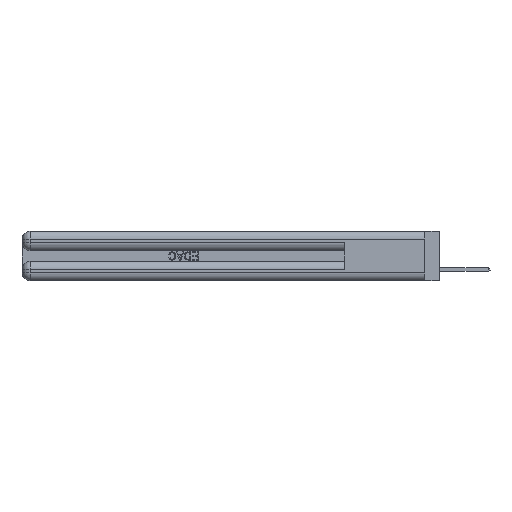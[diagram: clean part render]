
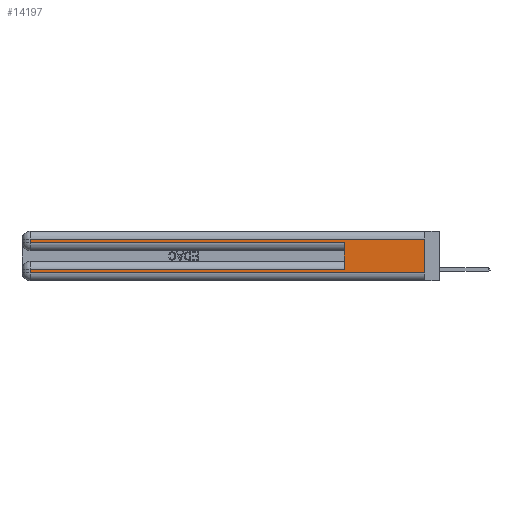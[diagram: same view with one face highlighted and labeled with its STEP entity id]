
A CAD part, left-side view. The second image highlights one B-rep face of the part: STEP entity #14197.
In plain terms, the highlighted planar face has unit normal (-1, 0, 0).
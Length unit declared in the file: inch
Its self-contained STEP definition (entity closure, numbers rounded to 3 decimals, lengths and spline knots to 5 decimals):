
#146 = EDGE_CURVE ( 'NONE', #34508, #25127, #3830, .T. ) ;
#267 = FACE_OUTER_BOUND ( 'NONE', #14080, .T. ) ;
#1153 = EDGE_CURVE ( 'NONE', #34851, #18567, #18973, .T. ) ;
#1823 = CARTESIAN_POINT ( 'NONE',  ( 0., 0., 0.31 ) ) ;
#2283 = CARTESIAN_POINT ( 'NONE',  ( 0., 0., 0.37 ) ) ;
#3098 = CARTESIAN_POINT ( 'NONE',  ( 0., 2.94, 0.06 ) ) ;
#3830 = LINE ( 'NONE', #24998, #38148 ) ;
#3988 = LINE ( 'NONE', #23489, #22519 ) ;
#4691 = ORIENTED_EDGE ( 'NONE', *, *, #10071, .T. ) ;
#5252 = VECTOR ( 'NONE', #17606, 39.37008 ) ;
#5422 = LINE ( 'NONE', #22631, #32078 ) ;
#6805 = CARTESIAN_POINT ( 'NONE',  ( 0., 0., 0.06 ) ) ;
#6834 = CARTESIAN_POINT ( 'NONE',  ( 0., 0., 0.37 ) ) ;
#7089 = LINE ( 'NONE', #20087, #37565 ) ;
#7390 = VERTEX_POINT ( 'NONE', #17802 ) ;
#8117 = DIRECTION ( 'NONE',  ( 0., 0., -1. ) ) ;
#8640 = ORIENTED_EDGE ( 'NONE', *, *, #18666, .F. ) ;
#10043 = VERTEX_POINT ( 'NONE', #35858 ) ;
#10071 = EDGE_CURVE ( 'NONE', #25127, #26792, #26643, .T. ) ;
#11554 = ORIENTED_EDGE ( 'NONE', *, *, #20790, .T. ) ;
#12254 = VERTEX_POINT ( 'NONE', #19260 ) ;
#12385 = CARTESIAN_POINT ( 'NONE',  ( 0., 2.94, 0.285 ) ) ;
#13328 = DIRECTION ( 'NONE',  ( 0., 1., 0. ) ) ;
#14080 = EDGE_LOOP ( 'NONE', ( #8640, #29875, #4691, #33569, #20254, #11554, #17339, #21712 ) ) ;
#14197 = ADVANCED_FACE ( 'NONE', ( #267 ), #20209, .F. ) ;
#17339 = ORIENTED_EDGE ( 'NONE', *, *, #24654, .T. ) ;
#17606 = DIRECTION ( 'NONE',  ( 0., 0., -1. ) ) ;
#17802 = CARTESIAN_POINT ( 'NONE',  ( 0., 0.6, 0.285 ) ) ;
#17845 = CARTESIAN_POINT ( 'NONE',  ( 0., 0., 0.085 ) ) ;
#18298 = VECTOR ( 'NONE', #38304, 39.37008 ) ;
#18567 = VERTEX_POINT ( 'NONE', #6805 ) ;
#18593 = DIRECTION ( 'NONE',  ( 0., 0., -1. ) ) ;
#18666 = EDGE_CURVE ( 'NONE', #34508, #18567, #25720, .T. ) ;
#18973 = LINE ( 'NONE', #37427, #21849 ) ;
#19260 = CARTESIAN_POINT ( 'NONE',  ( 0., 0.6, 0.085 ) ) ;
#19710 = DIRECTION ( 'NONE',  ( 0., 0., 1. ) ) ;
#20087 = CARTESIAN_POINT ( 'NONE',  ( 0., 2.94, 0.37 ) ) ;
#20209 = PLANE ( 'NONE',  #24529 ) ;
#20254 = ORIENTED_EDGE ( 'NONE', *, *, #37326, .F. ) ;
#20790 = EDGE_CURVE ( 'NONE', #12254, #10043, #26467, .T. ) ;
#21712 = ORIENTED_EDGE ( 'NONE', *, *, #1153, .T. ) ;
#21832 = VECTOR ( 'NONE', #18593, 39.37008 ) ;
#21849 = VECTOR ( 'NONE', #34229, 39.37008 ) ;
#22519 = VECTOR ( 'NONE', #35354, 39.37008 ) ;
#22631 = CARTESIAN_POINT ( 'NONE',  ( 0., 0.6, 0.145 ) ) ;
#23489 = CARTESIAN_POINT ( 'NONE',  ( 0., 0., 0.285 ) ) ;
#24529 = AXIS2_PLACEMENT_3D ( 'NONE', #2283, #38726, #8117 ) ;
#24654 = EDGE_CURVE ( 'NONE', #10043, #34851, #7089, .T. ) ;
#24998 = CARTESIAN_POINT ( 'NONE',  ( 0., 0., 0.31 ) ) ;
#25127 = VERTEX_POINT ( 'NONE', #26168 ) ;
#25720 = LINE ( 'NONE', #6834, #21832 ) ;
#26168 = CARTESIAN_POINT ( 'NONE',  ( 0., 2.94, 0.31 ) ) ;
#26467 = LINE ( 'NONE', #17845, #18298 ) ;
#26643 = LINE ( 'NONE', #38523, #5252 ) ;
#26792 = VERTEX_POINT ( 'NONE', #12385 ) ;
#28453 = EDGE_CURVE ( 'NONE', #26792, #7390, #3988, .T. ) ;
#29875 = ORIENTED_EDGE ( 'NONE', *, *, #146, .T. ) ;
#32078 = VECTOR ( 'NONE', #19710, 39.37008 ) ;
#33569 = ORIENTED_EDGE ( 'NONE', *, *, #28453, .T. ) ;
#34229 = DIRECTION ( 'NONE',  ( 0., -1., 0. ) ) ;
#34508 = VERTEX_POINT ( 'NONE', #1823 ) ;
#34851 = VERTEX_POINT ( 'NONE', #3098 ) ;
#35354 = DIRECTION ( 'NONE',  ( 0., -1., 0. ) ) ;
#35670 = DIRECTION ( 'NONE',  ( 0., 0., -1. ) ) ;
#35858 = CARTESIAN_POINT ( 'NONE',  ( 0., 2.94, 0.085 ) ) ;
#37326 = EDGE_CURVE ( 'NONE', #12254, #7390, #5422, .T. ) ;
#37427 = CARTESIAN_POINT ( 'NONE',  ( 0., 0., 0.06 ) ) ;
#37565 = VECTOR ( 'NONE', #35670, 39.37008 ) ;
#38148 = VECTOR ( 'NONE', #13328, 39.37008 ) ;
#38304 = DIRECTION ( 'NONE',  ( 0., 1., 0. ) ) ;
#38523 = CARTESIAN_POINT ( 'NONE',  ( 0., 2.94, 0.37 ) ) ;
#38726 = DIRECTION ( 'NONE',  ( 1., 0., 0. ) ) ;
